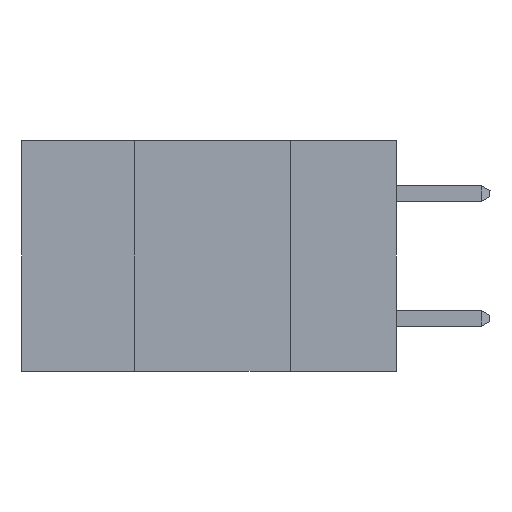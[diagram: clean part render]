
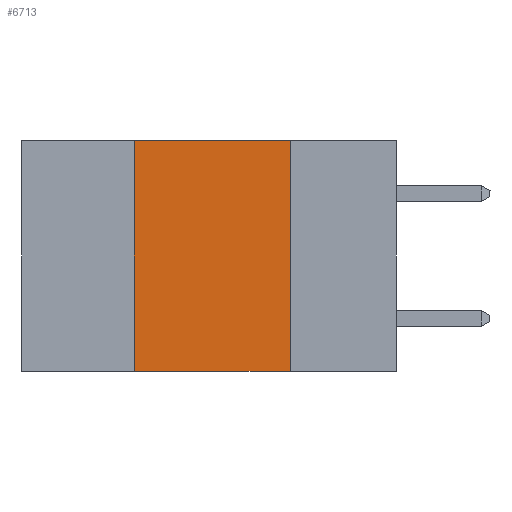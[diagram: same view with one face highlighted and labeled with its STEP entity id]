
A CAD part, left-side view. The second image highlights one B-rep face of the part: STEP entity #6713.
In plain terms, the highlighted planar face has unit normal (-1, 0, 0).
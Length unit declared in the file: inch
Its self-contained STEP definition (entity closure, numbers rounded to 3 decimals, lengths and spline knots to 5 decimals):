
#51 = DIRECTION ( 'NONE',  ( 0., 0., 1. ) ) ;
#239 = CARTESIAN_POINT ( 'NONE',  ( 0., 0.42, 0. ) ) ;
#331 = PLANE ( 'NONE',  #9130 ) ;
#973 = DIRECTION ( 'NONE',  ( 0., -1., 0. ) ) ;
#1468 = VERTEX_POINT ( 'NONE', #4953 ) ;
#1550 = VERTEX_POINT ( 'NONE', #239 ) ;
#1711 = VECTOR ( 'NONE', #6007, 39.37008 ) ;
#1871 = CARTESIAN_POINT ( 'NONE',  ( 0., 0.6, 0. ) ) ;
#2056 = EDGE_CURVE ( 'NONE', #3663, #8788, #4980, .T. ) ;
#2540 = CARTESIAN_POINT ( 'NONE',  ( 0., 0.42, 0. ) ) ;
#2952 = ORIENTED_EDGE ( 'NONE', *, *, #4186, .F. ) ;
#3093 = EDGE_LOOP ( 'NONE', ( #5939, #2952, #7277, #7569 ) ) ;
#3509 = CARTESIAN_POINT ( 'NONE',  ( 0., 0.17, 0. ) ) ;
#3663 = VERTEX_POINT ( 'NONE', #9715 ) ;
#3682 = VECTOR ( 'NONE', #973, 39.37008 ) ;
#4186 = EDGE_CURVE ( 'NONE', #1550, #3663, #8090, .T. ) ;
#4953 = CARTESIAN_POINT ( 'NONE',  ( 0., 0.42, -0.37 ) ) ;
#4980 = LINE ( 'NONE', #3509, #6666 ) ;
#5252 = CARTESIAN_POINT ( 'NONE',  ( 0., 0.17, -0.37 ) ) ;
#5319 = DIRECTION ( 'NONE',  ( 0., 0., -1. ) ) ;
#5889 = CARTESIAN_POINT ( 'NONE',  ( 0., 0.6, -0.37 ) ) ;
#5939 = ORIENTED_EDGE ( 'NONE', *, *, #2056, .F. ) ;
#6007 = DIRECTION ( 'NONE',  ( 0., -1., 0. ) ) ;
#6067 = DIRECTION ( 'NONE',  ( 0., 0., -1. ) ) ;
#6666 = VECTOR ( 'NONE', #5319, 39.37008 ) ;
#6713 = ADVANCED_FACE ( 'NONE', ( #8540 ), #331, .F. ) ;
#7277 = ORIENTED_EDGE ( 'NONE', *, *, #9949, .F. ) ;
#7569 = ORIENTED_EDGE ( 'NONE', *, *, #9344, .T. ) ;
#7689 = DIRECTION ( 'NONE',  ( 1., 0., 0. ) ) ;
#8090 = LINE ( 'NONE', #1871, #3682 ) ;
#8141 = VECTOR ( 'NONE', #51, 39.37008 ) ;
#8394 = LINE ( 'NONE', #2540, #8141 ) ;
#8540 = FACE_OUTER_BOUND ( 'NONE', #3093, .T. ) ;
#8788 = VERTEX_POINT ( 'NONE', #5252 ) ;
#9130 = AXIS2_PLACEMENT_3D ( 'NONE', #9489, #7689, #6067 ) ;
#9344 = EDGE_CURVE ( 'NONE', #1468, #8788, #9810, .T. ) ;
#9489 = CARTESIAN_POINT ( 'NONE',  ( 0., 0.6, 0. ) ) ;
#9715 = CARTESIAN_POINT ( 'NONE',  ( 0., 0.17, 0. ) ) ;
#9810 = LINE ( 'NONE', #5889, #1711 ) ;
#9949 = EDGE_CURVE ( 'NONE', #1468, #1550, #8394, .T. ) ;
